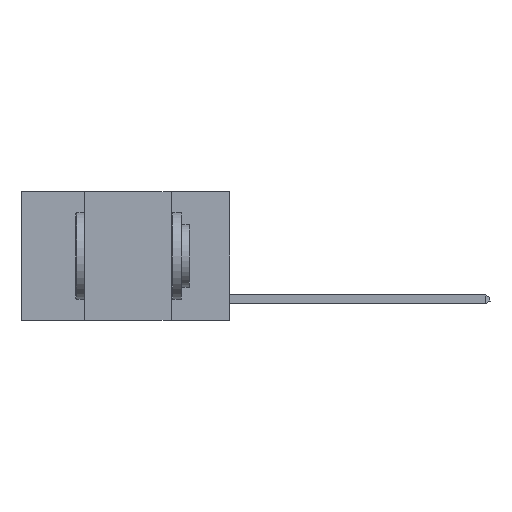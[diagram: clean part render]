
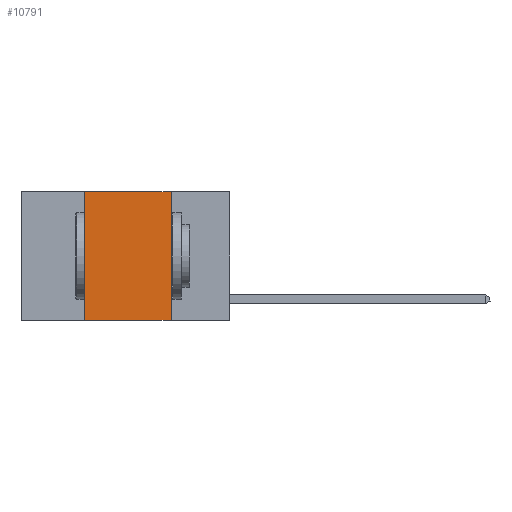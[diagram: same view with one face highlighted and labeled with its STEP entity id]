
A CAD part, left-side view. The second image highlights one B-rep face of the part: STEP entity #10791.
In plain terms, the highlighted planar face has unit normal (-1, 0, 0).
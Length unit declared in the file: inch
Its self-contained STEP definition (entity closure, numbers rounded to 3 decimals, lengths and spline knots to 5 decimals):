
#32 = ORIENTED_EDGE ( 'NONE', *, *, #9059, .F. ) ;
#100 = VECTOR ( 'NONE', #16668, 39.37008 ) ;
#875 = LINE ( 'NONE', #5009, #17013 ) ;
#1724 = AXIS2_PLACEMENT_3D ( 'NONE', #10179, #16843, #9914 ) ;
#1767 = LINE ( 'NONE', #5980, #14071 ) ;
#2016 = VERTEX_POINT ( 'NONE', #3889 ) ;
#2250 = EDGE_LOOP ( 'NONE', ( #32, #2861, #15974, #15444 ) ) ;
#2861 = ORIENTED_EDGE ( 'NONE', *, *, #4230, .F. ) ;
#3645 = EDGE_CURVE ( 'NONE', #12511, #12838, #12065, .T. ) ;
#3889 = CARTESIAN_POINT ( 'NONE',  ( 0., 0.17, 0. ) ) ;
#4230 = EDGE_CURVE ( 'NONE', #12838, #2016, #1767, .T. ) ;
#4833 = FACE_OUTER_BOUND ( 'NONE', #2250, .T. ) ;
#5009 = CARTESIAN_POINT ( 'NONE',  ( 0., 0.17, 0. ) ) ;
#5153 = CARTESIAN_POINT ( 'NONE',  ( 0., 0.6, -0.37 ) ) ;
#5980 = CARTESIAN_POINT ( 'NONE',  ( 0., 0.6, 0. ) ) ;
#6032 = PLANE ( 'NONE',  #1724 ) ;
#6789 = DIRECTION ( 'NONE',  ( 0., 0., 1. ) ) ;
#7484 = CARTESIAN_POINT ( 'NONE',  ( 0., 0.42, 0. ) ) ;
#7643 = LINE ( 'NONE', #5153, #100 ) ;
#8305 = DIRECTION ( 'NONE',  ( 0., -1., 0. ) ) ;
#9059 = EDGE_CURVE ( 'NONE', #2016, #15702, #875, .T. ) ;
#9914 = DIRECTION ( 'NONE',  ( 0., 0., -1. ) ) ;
#10179 = CARTESIAN_POINT ( 'NONE',  ( 0., 0.6, 0. ) ) ;
#10791 = ADVANCED_FACE ( 'NONE', ( #4833 ), #6032, .F. ) ;
#11968 = CARTESIAN_POINT ( 'NONE',  ( 0., 0.17, -0.37 ) ) ;
#11981 = CARTESIAN_POINT ( 'NONE',  ( 0., 0.42, -0.37 ) ) ;
#12065 = LINE ( 'NONE', #13483, #13011 ) ;
#12511 = VERTEX_POINT ( 'NONE', #11981 ) ;
#12787 = EDGE_CURVE ( 'NONE', #12511, #15702, #7643, .T. ) ;
#12838 = VERTEX_POINT ( 'NONE', #7484 ) ;
#13011 = VECTOR ( 'NONE', #6789, 39.37008 ) ;
#13483 = CARTESIAN_POINT ( 'NONE',  ( 0., 0.42, 0. ) ) ;
#14071 = VECTOR ( 'NONE', #8305, 39.37008 ) ;
#15444 = ORIENTED_EDGE ( 'NONE', *, *, #12787, .T. ) ;
#15702 = VERTEX_POINT ( 'NONE', #11968 ) ;
#15974 = ORIENTED_EDGE ( 'NONE', *, *, #3645, .F. ) ;
#16531 = DIRECTION ( 'NONE',  ( 0., 0., -1. ) ) ;
#16668 = DIRECTION ( 'NONE',  ( 0., -1., 0. ) ) ;
#16843 = DIRECTION ( 'NONE',  ( 1., 0., 0. ) ) ;
#17013 = VECTOR ( 'NONE', #16531, 39.37008 ) ;
